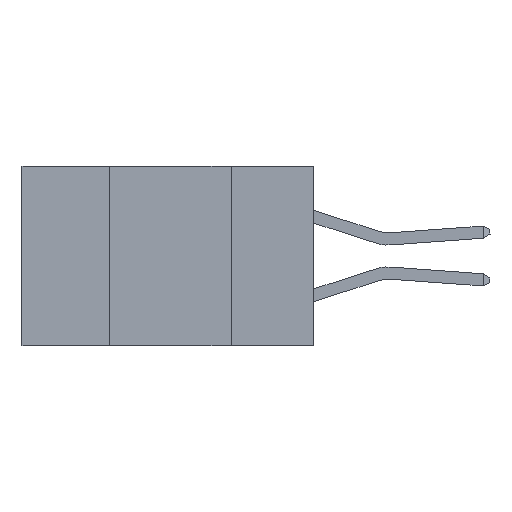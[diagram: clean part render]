
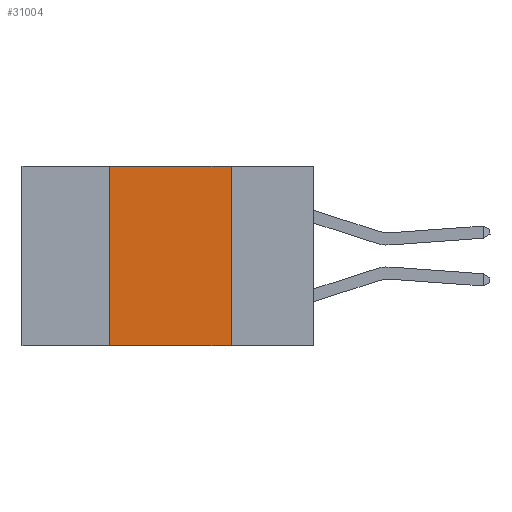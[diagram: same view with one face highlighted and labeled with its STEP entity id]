
A CAD part, left-side view. The second image highlights one B-rep face of the part: STEP entity #31004.
In plain terms, the highlighted planar face has unit normal (-1, 0, 0).
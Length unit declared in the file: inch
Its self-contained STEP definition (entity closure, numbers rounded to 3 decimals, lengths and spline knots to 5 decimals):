
#37 = LINE ( 'NONE', #32551, #16586 ) ;
#544 = CARTESIAN_POINT ( 'NONE',  ( 0., 0.6, 0. ) ) ;
#1013 = VERTEX_POINT ( 'NONE', #19194 ) ;
#1124 = PLANE ( 'NONE',  #3038 ) ;
#1472 = DIRECTION ( 'NONE',  ( 1., 0., 0. ) ) ;
#2833 = CARTESIAN_POINT ( 'NONE',  ( 0., 0.42, -0.37 ) ) ;
#3038 = AXIS2_PLACEMENT_3D ( 'NONE', #14900, #1472, #27997 ) ;
#3228 = VECTOR ( 'NONE', #8329, 39.37008 ) ;
#3992 = CARTESIAN_POINT ( 'NONE',  ( 0., 0.17, 0. ) ) ;
#4115 = LINE ( 'NONE', #22687, #26686 ) ;
#5318 = ORIENTED_EDGE ( 'NONE', *, *, #28026, .F. ) ;
#6016 = LINE ( 'NONE', #544, #3228 ) ;
#6583 = DIRECTION ( 'NONE',  ( 0., 0., 1. ) ) ;
#7467 = DIRECTION ( 'NONE',  ( 0., -1., 0. ) ) ;
#7519 = VECTOR ( 'NONE', #7467, 39.37008 ) ;
#8329 = DIRECTION ( 'NONE',  ( 0., -1., 0. ) ) ;
#9855 = VERTEX_POINT ( 'NONE', #25538 ) ;
#11555 = ORIENTED_EDGE ( 'NONE', *, *, #22896, .F. ) ;
#11900 = EDGE_CURVE ( 'NONE', #9855, #22203, #6016, .T. ) ;
#12936 = LINE ( 'NONE', #31682, #7519 ) ;
#14900 = CARTESIAN_POINT ( 'NONE',  ( 0., 0.6, 0. ) ) ;
#16586 = VECTOR ( 'NONE', #27261, 39.37008 ) ;
#19194 = CARTESIAN_POINT ( 'NONE',  ( 0., 0.17, -0.37 ) ) ;
#22203 = VERTEX_POINT ( 'NONE', #3992 ) ;
#22687 = CARTESIAN_POINT ( 'NONE',  ( 0., 0.42, 0. ) ) ;
#22896 = EDGE_CURVE ( 'NONE', #22203, #1013, #37, .T. ) ;
#23616 = ORIENTED_EDGE ( 'NONE', *, *, #11900, .F. ) ;
#24189 = EDGE_CURVE ( 'NONE', #30405, #1013, #12936, .T. ) ;
#25271 = ORIENTED_EDGE ( 'NONE', *, *, #24189, .T. ) ;
#25538 = CARTESIAN_POINT ( 'NONE',  ( 0., 0.42, 0. ) ) ;
#26686 = VECTOR ( 'NONE', #6583, 39.37008 ) ;
#27261 = DIRECTION ( 'NONE',  ( 0., 0., -1. ) ) ;
#27997 = DIRECTION ( 'NONE',  ( 0., 0., -1. ) ) ;
#28026 = EDGE_CURVE ( 'NONE', #30405, #9855, #4115, .T. ) ;
#28511 = FACE_OUTER_BOUND ( 'NONE', #33673, .T. ) ;
#30405 = VERTEX_POINT ( 'NONE', #2833 ) ;
#31004 = ADVANCED_FACE ( 'NONE', ( #28511 ), #1124, .F. ) ;
#31682 = CARTESIAN_POINT ( 'NONE',  ( 0., 0.6, -0.37 ) ) ;
#32551 = CARTESIAN_POINT ( 'NONE',  ( 0., 0.17, 0. ) ) ;
#33673 = EDGE_LOOP ( 'NONE', ( #11555, #23616, #5318, #25271 ) ) ;
